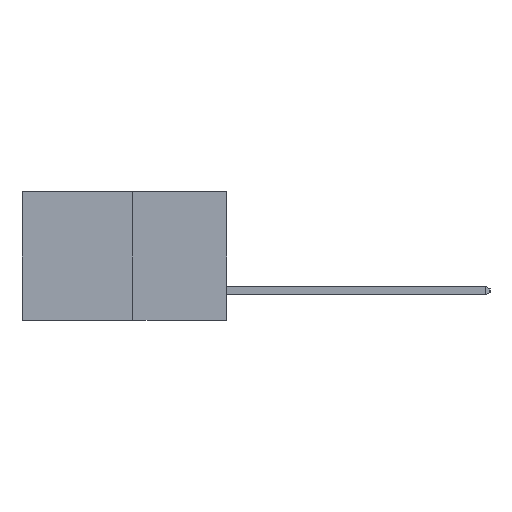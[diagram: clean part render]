
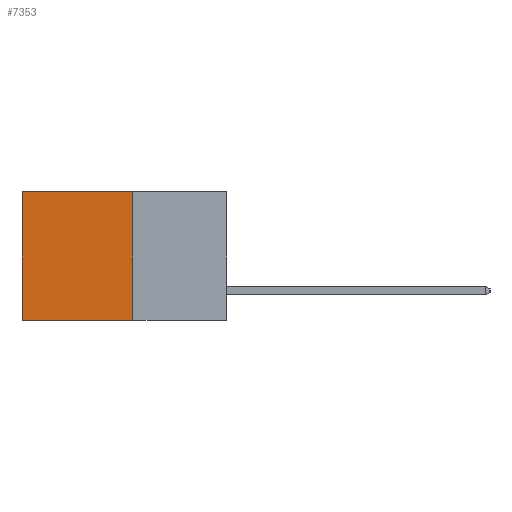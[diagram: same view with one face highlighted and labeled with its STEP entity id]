
A CAD part, left-side view. The second image highlights one B-rep face of the part: STEP entity #7353.
In plain terms, the highlighted planar face has unit normal (-1, 0, 0).
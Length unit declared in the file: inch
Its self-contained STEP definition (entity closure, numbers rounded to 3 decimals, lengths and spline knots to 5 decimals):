
#594 = VERTEX_POINT ( 'NONE', #14049 ) ;
#1568 = ORIENTED_EDGE ( 'NONE', *, *, #9617, .F. ) ;
#1802 = PLANE ( 'NONE',  #15663 ) ;
#2046 = EDGE_CURVE ( 'NONE', #23094, #13836, #17428, .T. ) ;
#2467 = VECTOR ( 'NONE', #3686, 39.37008 ) ;
#2602 = ORIENTED_EDGE ( 'NONE', *, *, #21712, .T. ) ;
#2969 = VECTOR ( 'NONE', #13438, 39.37008 ) ;
#3203 = CARTESIAN_POINT ( 'NONE',  ( 0.277, 0.27, 0. ) ) ;
#3686 = DIRECTION ( 'NONE',  ( 0., 0., -1. ) ) ;
#4040 = EDGE_CURVE ( 'NONE', #22063, #594, #12653, .T. ) ;
#5580 = DIRECTION ( 'NONE',  ( 0., 0., -1. ) ) ;
#5589 = ORIENTED_EDGE ( 'NONE', *, *, #4040, .T. ) ;
#7353 = ADVANCED_FACE ( 'NONE', ( #15820 ), #1802, .F. ) ;
#7464 = CARTESIAN_POINT ( 'NONE',  ( 0.277, 0.27, -0.37 ) ) ;
#7726 = ORIENTED_EDGE ( 'NONE', *, *, #2046, .F. ) ;
#9617 = EDGE_CURVE ( 'NONE', #13836, #594, #20985, .T. ) ;
#9661 = CARTESIAN_POINT ( 'NONE',  ( 0.277, 0.59, 0. ) ) ;
#9912 = VECTOR ( 'NONE', #14086, 39.37008 ) ;
#11576 = VECTOR ( 'NONE', #16963, 39.37008 ) ;
#11610 = CARTESIAN_POINT ( 'NONE',  ( 0.277, 0.27, -0.37 ) ) ;
#12653 = LINE ( 'NONE', #13025, #2969 ) ;
#13025 = CARTESIAN_POINT ( 'NONE',  ( 0.277, 0.59, -0.37 ) ) ;
#13438 = DIRECTION ( 'NONE',  ( 0., 0., -1. ) ) ;
#13836 = VERTEX_POINT ( 'NONE', #22343 ) ;
#14049 = CARTESIAN_POINT ( 'NONE',  ( 0.277, 0.59, -0.37 ) ) ;
#14086 = DIRECTION ( 'NONE',  ( 0., 1., 0. ) ) ;
#15663 = AXIS2_PLACEMENT_3D ( 'NONE', #23316, #16314, #5580 ) ;
#15820 = FACE_OUTER_BOUND ( 'NONE', #16978, .T. ) ;
#16314 = DIRECTION ( 'NONE',  ( 1., 0., 0. ) ) ;
#16517 = CARTESIAN_POINT ( 'NONE',  ( 0.277, 0.27, 0. ) ) ;
#16963 = DIRECTION ( 'NONE',  ( 0., 1., 0. ) ) ;
#16978 = EDGE_LOOP ( 'NONE', ( #5589, #1568, #7726, #2602 ) ) ;
#17428 = LINE ( 'NONE', #7464, #2467 ) ;
#19344 = LINE ( 'NONE', #3203, #9912 ) ;
#20985 = LINE ( 'NONE', #11610, #11576 ) ;
#21712 = EDGE_CURVE ( 'NONE', #23094, #22063, #19344, .T. ) ;
#22063 = VERTEX_POINT ( 'NONE', #9661 ) ;
#22343 = CARTESIAN_POINT ( 'NONE',  ( 0.277, 0.27, -0.37 ) ) ;
#23094 = VERTEX_POINT ( 'NONE', #16517 ) ;
#23316 = CARTESIAN_POINT ( 'NONE',  ( 0.277, 0.27, -0.37 ) ) ;
